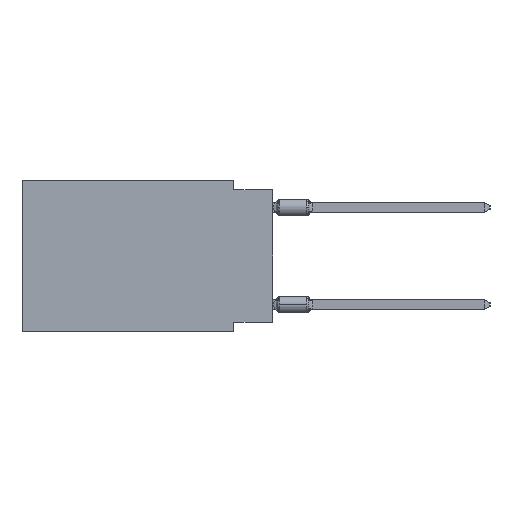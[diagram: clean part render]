
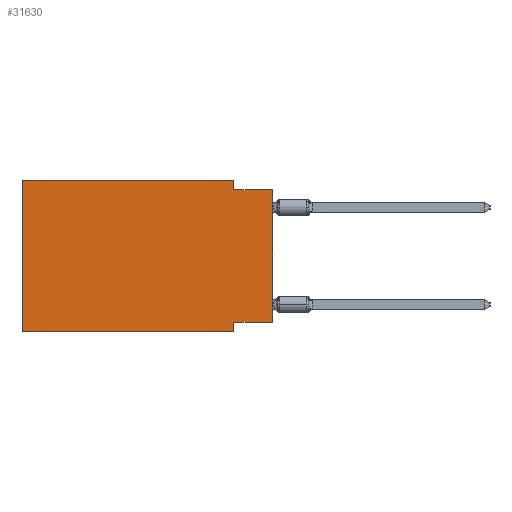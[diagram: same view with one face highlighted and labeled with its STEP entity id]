
A CAD part, left-side view. The second image highlights one B-rep face of the part: STEP entity #31630.
In plain terms, the highlighted planar face has unit normal (-1, 0, 0).
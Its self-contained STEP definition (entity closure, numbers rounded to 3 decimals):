
#2512 = VECTOR ( 'NONE', #23208, 1000. ) ;
#3845 = VERTEX_POINT ( 'NONE', #50409 ) ;
#5783 = VERTEX_POINT ( 'NONE', #33541 ) ;
#7777 = DIRECTION ( 'NONE',  ( 0., -1., 0. ) ) ;
#9184 = VECTOR ( 'NONE', #61258, 1000. ) ;
#9248 = ORIENTED_EDGE ( 'NONE', *, *, #14224, .F. ) ;
#10088 = EDGE_LOOP ( 'NONE', ( #25384, #9248, #40404, #24899, #57477, #19487, #47114, #29945 ) ) ;
#11232 = DIRECTION ( 'NONE',  ( 0., 0., 1. ) ) ;
#11868 = CARTESIAN_POINT ( 'NONE',  ( 0., 16.383, 0. ) ) ;
#12603 = LINE ( 'NONE', #23529, #53430 ) ;
#12620 = CARTESIAN_POINT ( 'NONE',  ( 0., 0., -0.635 ) ) ;
#13371 = VERTEX_POINT ( 'NONE', #62903 ) ;
#14224 = EDGE_CURVE ( 'NONE', #5783, #52951, #65403, .T. ) ;
#16975 = EDGE_CURVE ( 'NONE', #62051, #13371, #51592, .T. ) ;
#17154 = PLANE ( 'NONE',  #34040 ) ;
#17675 = DIRECTION ( 'NONE',  ( 0., 0., 1. ) ) ;
#19264 = VECTOR ( 'NONE', #11232, 1000. ) ;
#19487 = ORIENTED_EDGE ( 'NONE', *, *, #55181, .T. ) ;
#20022 = VERTEX_POINT ( 'NONE', #48054 ) ;
#21918 = EDGE_CURVE ( 'NONE', #64784, #20022, #41080, .T. ) ;
#23208 = DIRECTION ( 'NONE',  ( 0., 0., -1. ) ) ;
#23529 = CARTESIAN_POINT ( 'NONE',  ( 0., 16.383, -9.906 ) ) ;
#24899 = ORIENTED_EDGE ( 'NONE', *, *, #16975, .F. ) ;
#25384 = ORIENTED_EDGE ( 'NONE', *, *, #47513, .T. ) ;
#26550 = EDGE_CURVE ( 'NONE', #30952, #62051, #26933, .T. ) ;
#26933 = LINE ( 'NONE', #11868, #32263 ) ;
#27505 = VECTOR ( 'NONE', #59616, 1000. ) ;
#29009 = CARTESIAN_POINT ( 'NONE',  ( 0., 2.54, 0. ) ) ;
#29945 = ORIENTED_EDGE ( 'NONE', *, *, #39326, .F. ) ;
#30186 = CARTESIAN_POINT ( 'NONE',  ( 0., 16.383, 0. ) ) ;
#30680 = CARTESIAN_POINT ( 'NONE',  ( 0., 16.383, -9.906 ) ) ;
#30952 = VERTEX_POINT ( 'NONE', #30680 ) ;
#31630 = ADVANCED_FACE ( 'NONE', ( #47914 ), #17154, .F. ) ;
#32263 = VECTOR ( 'NONE', #17675, 1000. ) ;
#32847 = DIRECTION ( 'NONE',  ( 0., 0., -1. ) ) ;
#33466 = LINE ( 'NONE', #29009, #2512 ) ;
#33541 = CARTESIAN_POINT ( 'NONE',  ( 0., 2.54, -0.635 ) ) ;
#33853 = CARTESIAN_POINT ( 'NONE',  ( 0., 16.383, 0. ) ) ;
#34040 = AXIS2_PLACEMENT_3D ( 'NONE', #33853, #37991, #32847 ) ;
#36204 = DIRECTION ( 'NONE',  ( 0., -1., 0. ) ) ;
#37212 = CARTESIAN_POINT ( 'NONE',  ( 0., 0., 0. ) ) ;
#37991 = DIRECTION ( 'NONE',  ( 1., 0., 0. ) ) ;
#38348 = VECTOR ( 'NONE', #49304, 1000. ) ;
#39326 = EDGE_CURVE ( 'NONE', #3845, #64784, #40383, .T. ) ;
#40383 = LINE ( 'NONE', #61244, #38348 ) ;
#40404 = ORIENTED_EDGE ( 'NONE', *, *, #59716, .F. ) ;
#41080 = LINE ( 'NONE', #45865, #9184 ) ;
#45865 = CARTESIAN_POINT ( 'NONE',  ( 0., 2.54, -9.906 ) ) ;
#47114 = ORIENTED_EDGE ( 'NONE', *, *, #21918, .F. ) ;
#47513 = EDGE_CURVE ( 'NONE', #3845, #52951, #63218, .T. ) ;
#47914 = FACE_OUTER_BOUND ( 'NONE', #10088, .T. ) ;
#48054 = CARTESIAN_POINT ( 'NONE',  ( 0., 2.54, -9.906 ) ) ;
#49304 = DIRECTION ( 'NONE',  ( 0., 1., 0. ) ) ;
#50409 = CARTESIAN_POINT ( 'NONE',  ( 0., 0., -9.271 ) ) ;
#51592 = LINE ( 'NONE', #51947, #56929 ) ;
#51947 = CARTESIAN_POINT ( 'NONE',  ( 0., 16.383, 0. ) ) ;
#52951 = VERTEX_POINT ( 'NONE', #12620 ) ;
#53430 = VECTOR ( 'NONE', #7777, 1000. ) ;
#55145 = CARTESIAN_POINT ( 'NONE',  ( 0., 0., -0.635 ) ) ;
#55181 = EDGE_CURVE ( 'NONE', #30952, #20022, #12603, .T. ) ;
#56929 = VECTOR ( 'NONE', #36204, 1000. ) ;
#57389 = CARTESIAN_POINT ( 'NONE',  ( 0., 2.54, -9.271 ) ) ;
#57477 = ORIENTED_EDGE ( 'NONE', *, *, #26550, .F. ) ;
#59616 = DIRECTION ( 'NONE',  ( 0., -1., 0. ) ) ;
#59716 = EDGE_CURVE ( 'NONE', #13371, #5783, #33466, .T. ) ;
#61244 = CARTESIAN_POINT ( 'NONE',  ( 0., 0., -9.271 ) ) ;
#61258 = DIRECTION ( 'NONE',  ( 0., 0., -1. ) ) ;
#62051 = VERTEX_POINT ( 'NONE', #30186 ) ;
#62903 = CARTESIAN_POINT ( 'NONE',  ( 0., 2.54, 0. ) ) ;
#63218 = LINE ( 'NONE', #37212, #19264 ) ;
#64784 = VERTEX_POINT ( 'NONE', #57389 ) ;
#65403 = LINE ( 'NONE', #55145, #27505 ) ;
